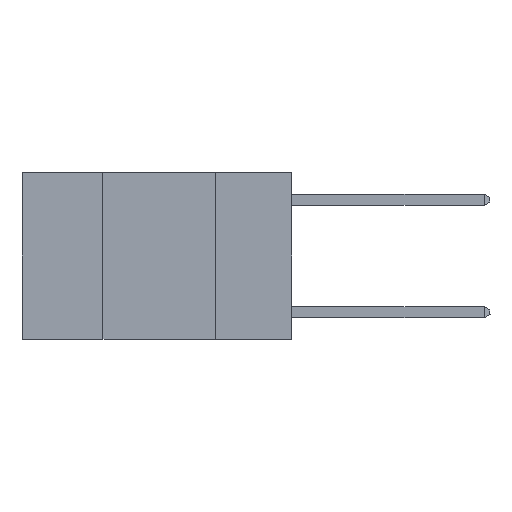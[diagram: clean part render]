
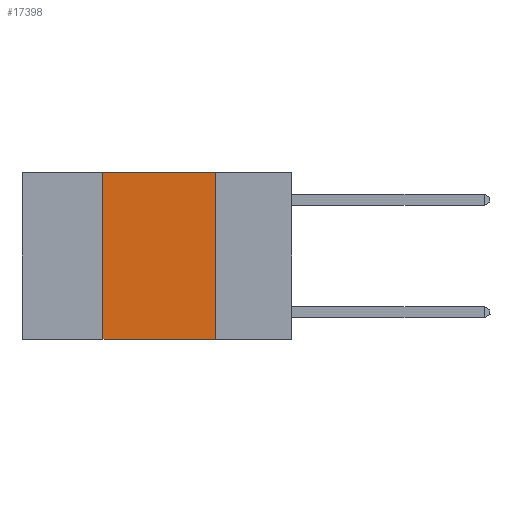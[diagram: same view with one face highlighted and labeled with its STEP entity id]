
A CAD part, left-side view. The second image highlights one B-rep face of the part: STEP entity #17398.
In plain terms, the highlighted planar face has unit normal (-1, 0, 0).
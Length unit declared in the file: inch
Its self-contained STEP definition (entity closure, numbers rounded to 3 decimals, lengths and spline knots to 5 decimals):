
#442 = DIRECTION ( 'NONE',  ( 0., 0., -1. ) ) ;
#573 = VERTEX_POINT ( 'NONE', #13804 ) ;
#726 = DIRECTION ( 'NONE',  ( 0., -1., 0. ) ) ;
#874 = DIRECTION ( 'NONE',  ( 0., 0., 1. ) ) ;
#2659 = EDGE_CURVE ( 'NONE', #12579, #573, #5492, .T. ) ;
#3301 = CARTESIAN_POINT ( 'NONE',  ( 0., 0.17, 0. ) ) ;
#4402 = CARTESIAN_POINT ( 'NONE',  ( 0., 0.6, -0.37 ) ) ;
#4917 = VERTEX_POINT ( 'NONE', #15345 ) ;
#5081 = EDGE_CURVE ( 'NONE', #7892, #12579, #14172, .T. ) ;
#5203 = DIRECTION ( 'NONE',  ( 0., 0., -1. ) ) ;
#5492 = LINE ( 'NONE', #19669, #20339 ) ;
#5708 = CARTESIAN_POINT ( 'NONE',  ( 0., 0.42, 0. ) ) ;
#7892 = VERTEX_POINT ( 'NONE', #18005 ) ;
#7905 = ORIENTED_EDGE ( 'NONE', *, *, #11068, .F. ) ;
#8319 = CARTESIAN_POINT ( 'NONE',  ( 0., 0.42, 0. ) ) ;
#8553 = DIRECTION ( 'NONE',  ( 0., -1., 0. ) ) ;
#8611 = VECTOR ( 'NONE', #726, 39.37008 ) ;
#9202 = VECTOR ( 'NONE', #874, 39.37008 ) ;
#9408 = ORIENTED_EDGE ( 'NONE', *, *, #12774, .T. ) ;
#9785 = CARTESIAN_POINT ( 'NONE',  ( 0., 0.6, 0. ) ) ;
#11068 = EDGE_CURVE ( 'NONE', #573, #4917, #20581, .T. ) ;
#11696 = DIRECTION ( 'NONE',  ( 1., 0., 0. ) ) ;
#12579 = VERTEX_POINT ( 'NONE', #5708 ) ;
#12774 = EDGE_CURVE ( 'NONE', #7892, #4917, #22237, .T. ) ;
#13804 = CARTESIAN_POINT ( 'NONE',  ( 0., 0.17, 0. ) ) ;
#14172 = LINE ( 'NONE', #8319, #9202 ) ;
#14666 = ORIENTED_EDGE ( 'NONE', *, *, #2659, .F. ) ;
#15345 = CARTESIAN_POINT ( 'NONE',  ( 0., 0.17, -0.37 ) ) ;
#16282 = VECTOR ( 'NONE', #5203, 39.37008 ) ;
#17165 = PLANE ( 'NONE',  #18735 ) ;
#17398 = ADVANCED_FACE ( 'NONE', ( #19686 ), #17165, .F. ) ;
#18005 = CARTESIAN_POINT ( 'NONE',  ( 0., 0.42, -0.37 ) ) ;
#18123 = ORIENTED_EDGE ( 'NONE', *, *, #5081, .F. ) ;
#18735 = AXIS2_PLACEMENT_3D ( 'NONE', #9785, #11696, #442 ) ;
#19669 = CARTESIAN_POINT ( 'NONE',  ( 0., 0.6, 0. ) ) ;
#19686 = FACE_OUTER_BOUND ( 'NONE', #23749, .T. ) ;
#20339 = VECTOR ( 'NONE', #8553, 39.37008 ) ;
#20581 = LINE ( 'NONE', #3301, #16282 ) ;
#22237 = LINE ( 'NONE', #4402, #8611 ) ;
#23749 = EDGE_LOOP ( 'NONE', ( #7905, #14666, #18123, #9408 ) ) ;
